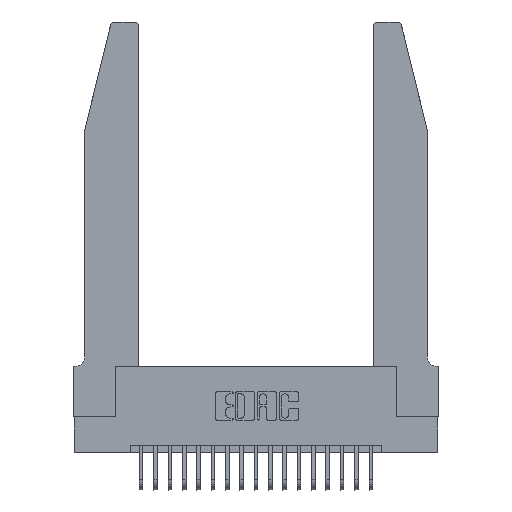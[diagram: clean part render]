
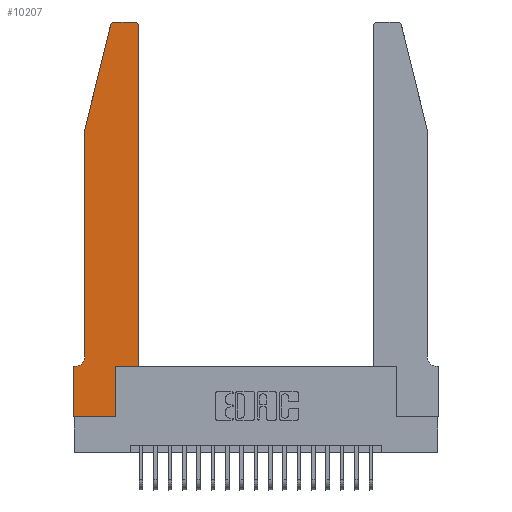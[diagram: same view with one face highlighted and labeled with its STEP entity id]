
A CAD part, top view. The second image highlights one B-rep face of the part: STEP entity #10207.
In plain terms, the highlighted planar face has unit normal (0, 0, 1).
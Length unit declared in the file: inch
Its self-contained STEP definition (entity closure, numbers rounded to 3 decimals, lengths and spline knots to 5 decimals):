
#33 = DIRECTION ( 'NONE',  ( 0., 0., -1. ) ) ;
#140 = LINE ( 'NONE', #16680, #13970 ) ;
#175 = ORIENTED_EDGE ( 'NONE', *, *, #2463, .T. ) ;
#192 = CARTESIAN_POINT ( 'NONE',  ( 0., 0., 0.37 ) ) ;
#350 = VERTEX_POINT ( 'NONE', #192 ) ;
#1004 = DIRECTION ( 'NONE',  ( 1., 0., 0. ) ) ;
#1523 = EDGE_CURVE ( 'NONE', #8714, #16386, #11315, .T. ) ;
#1580 = CARTESIAN_POINT ( 'NONE',  ( 0.0755, 0.42, 0.37 ) ) ;
#1600 = CARTESIAN_POINT ( 'NONE',  ( 0., 0.35, 0.37 ) ) ;
#1772 = VECTOR ( 'NONE', #22418, 39.37008 ) ;
#1988 = ORIENTED_EDGE ( 'NONE', *, *, #7056, .T. ) ;
#2077 = CIRCLE ( 'NONE', #5334, 0.07 ) ;
#2463 = EDGE_CURVE ( 'NONE', #16386, #350, #21253, .T. ) ;
#2477 = VECTOR ( 'NONE', #8777, 39.37008 ) ;
#2504 = ORIENTED_EDGE ( 'NONE', *, *, #20035, .T. ) ;
#3060 = EDGE_CURVE ( 'NONE', #12138, #10161, #10993, .T. ) ;
#3272 = EDGE_CURVE ( 'NONE', #13360, #10950, #6534, .T. ) ;
#3466 = CARTESIAN_POINT ( 'NONE',  ( 0., 0.35, 0.37 ) ) ;
#4598 = CARTESIAN_POINT ( 'NONE',  ( 0.2865, 0.35, 0.37 ) ) ;
#4652 = ORIENTED_EDGE ( 'NONE', *, *, #5797, .T. ) ;
#4899 = VECTOR ( 'NONE', #6230, 39.37008 ) ;
#5225 = ORIENTED_EDGE ( 'NONE', *, *, #17282, .T. ) ;
#5261 = DIRECTION ( 'NONE',  ( 0., 0., 1. ) ) ;
#5334 = AXIS2_PLACEMENT_3D ( 'NONE', #10839, #33, #12690 ) ;
#5691 = DIRECTION ( 'NONE',  ( -1., 0., 0. ) ) ;
#5749 = DIRECTION ( 'NONE',  ( 1., 0., 0. ) ) ;
#5797 = EDGE_CURVE ( 'NONE', #10161, #20009, #22704, .T. ) ;
#5810 = DIRECTION ( 'NONE',  ( 0., 0., 1. ) ) ;
#5892 = EDGE_LOOP ( 'NONE', ( #22410, #4652, #5225, #6139, #2504, #12326, #175, #20078, #11776, #21731, #1988, #7278 ) ) ;
#5941 = CARTESIAN_POINT ( 'NONE',  ( 0.4505, 0.35, 0.37 ) ) ;
#6001 = CARTESIAN_POINT ( 'NONE',  ( 0.0755, 2., 0.37 ) ) ;
#6014 = VECTOR ( 'NONE', #5691, 39.37008 ) ;
#6139 = ORIENTED_EDGE ( 'NONE', *, *, #14868, .T. ) ;
#6230 = DIRECTION ( 'NONE',  ( 0., 1., 0. ) ) ;
#6391 = CARTESIAN_POINT ( 'NONE',  ( 0.2865, 0., 0.37 ) ) ;
#6481 = CARTESIAN_POINT ( 'NONE',  ( 0.4505, 2.72, 0.37 ) ) ;
#6489 = CARTESIAN_POINT ( 'NONE',  ( 0.2605, 2.75, 0.37 ) ) ;
#6495 = VERTEX_POINT ( 'NONE', #6481 ) ;
#6534 = LINE ( 'NONE', #4598, #1772 ) ;
#7056 = EDGE_CURVE ( 'NONE', #10505, #6495, #19098, .T. ) ;
#7063 = VECTOR ( 'NONE', #22277, 39.37008 ) ;
#7187 = LINE ( 'NONE', #15875, #2477 ) ;
#7211 = AXIS2_PLACEMENT_3D ( 'NONE', #16465, #5810, #18267 ) ;
#7278 = ORIENTED_EDGE ( 'NONE', *, *, #14237, .T. ) ;
#7307 = VECTOR ( 'NONE', #5749, 39.37008 ) ;
#7722 = VERTEX_POINT ( 'NONE', #1580 ) ;
#8655 = CARTESIAN_POINT ( 'NONE',  ( 0.0755, 0.35, 0.37 ) ) ;
#8714 = VERTEX_POINT ( 'NONE', #11306 ) ;
#8777 = DIRECTION ( 'NONE',  ( 1., 0., 0. ) ) ;
#9510 = VECTOR ( 'NONE', #18959, 39.37008 ) ;
#10161 = VERTEX_POINT ( 'NONE', #22833 ) ;
#10207 = ADVANCED_FACE ( 'NONE', ( #20591 ), #14140, .T. ) ;
#10505 = VERTEX_POINT ( 'NONE', #5941 ) ;
#10839 = CARTESIAN_POINT ( 'NONE',  ( 0.0055, 0.42, 0.37 ) ) ;
#10887 = EDGE_CURVE ( 'NONE', #350, #13360, #7187, .T. ) ;
#10950 = VERTEX_POINT ( 'NONE', #12583 ) ;
#10993 = LINE ( 'NONE', #6489, #19346 ) ;
#11306 = CARTESIAN_POINT ( 'NONE',  ( 0.0055, 0.35, 0.37 ) ) ;
#11315 = LINE ( 'NONE', #8655, #6014 ) ;
#11752 = DIRECTION ( 'NONE',  ( 0., 0., 1. ) ) ;
#11776 = ORIENTED_EDGE ( 'NONE', *, *, #3272, .T. ) ;
#12138 = VERTEX_POINT ( 'NONE', #13473 ) ;
#12326 = ORIENTED_EDGE ( 'NONE', *, *, #1523, .T. ) ;
#12583 = CARTESIAN_POINT ( 'NONE',  ( 0.2865, 0.35, 0.37 ) ) ;
#12690 = DIRECTION ( 'NONE',  ( -1., 0., 0. ) ) ;
#13360 = VERTEX_POINT ( 'NONE', #6391 ) ;
#13473 = CARTESIAN_POINT ( 'NONE',  ( 0.4205, 2.75, 0.37 ) ) ;
#13708 = AXIS2_PLACEMENT_3D ( 'NONE', #22329, #11752, #1004 ) ;
#13970 = VECTOR ( 'NONE', #18398, 39.37008 ) ;
#14065 = CIRCLE ( 'NONE', #7211, 0.03 ) ;
#14140 = PLANE ( 'NONE',  #15374 ) ;
#14237 = EDGE_CURVE ( 'NONE', #6495, #12138, #14065, .T. ) ;
#14282 = LINE ( 'NONE', #22399, #9510 ) ;
#14563 = EDGE_CURVE ( 'NONE', #10950, #10505, #20403, .T. ) ;
#14868 = EDGE_CURVE ( 'NONE', #20848, #7722, #14282, .T. ) ;
#15374 = AXIS2_PLACEMENT_3D ( 'NONE', #3466, #5261, #17714 ) ;
#15875 = CARTESIAN_POINT ( 'NONE',  ( 0., 0., 0.37 ) ) ;
#16386 = VERTEX_POINT ( 'NONE', #1600 ) ;
#16397 = CARTESIAN_POINT ( 'NONE',  ( 0.4505, 0.35, 0.37 ) ) ;
#16465 = CARTESIAN_POINT ( 'NONE',  ( 0.4205, 2.72, 0.37 ) ) ;
#16680 = CARTESIAN_POINT ( 'NONE',  ( 0.0755, 2., 0.37 ) ) ;
#17282 = EDGE_CURVE ( 'NONE', #20009, #20848, #140, .T. ) ;
#17714 = DIRECTION ( 'NONE',  ( 1., 0., 0. ) ) ;
#18075 = DIRECTION ( 'NONE',  ( -1., 0., 0. ) ) ;
#18267 = DIRECTION ( 'NONE',  ( 1., 0., 0. ) ) ;
#18398 = DIRECTION ( 'NONE',  ( -0.239, -0.971, 0. ) ) ;
#18459 = CARTESIAN_POINT ( 'NONE',  ( 0.25487, 2.72718, 0.37 ) ) ;
#18959 = DIRECTION ( 'NONE',  ( 0., -1., 0. ) ) ;
#19098 = LINE ( 'NONE', #20360, #4899 ) ;
#19346 = VECTOR ( 'NONE', #18075, 39.37008 ) ;
#20009 = VERTEX_POINT ( 'NONE', #18459 ) ;
#20035 = EDGE_CURVE ( 'NONE', #7722, #8714, #2077, .T. ) ;
#20078 = ORIENTED_EDGE ( 'NONE', *, *, #10887, .T. ) ;
#20360 = CARTESIAN_POINT ( 'NONE',  ( 0.4505, 0.35, 0.37 ) ) ;
#20403 = LINE ( 'NONE', #16397, #7307 ) ;
#20533 = CARTESIAN_POINT ( 'NONE',  ( 0., 0., 0.37 ) ) ;
#20591 = FACE_OUTER_BOUND ( 'NONE', #5892, .T. ) ;
#20848 = VERTEX_POINT ( 'NONE', #6001 ) ;
#21253 = LINE ( 'NONE', #20533, #7063 ) ;
#21731 = ORIENTED_EDGE ( 'NONE', *, *, #14563, .T. ) ;
#22277 = DIRECTION ( 'NONE',  ( 0., -1., 0. ) ) ;
#22329 = CARTESIAN_POINT ( 'NONE',  ( 0.284, 2.72, 0.37 ) ) ;
#22399 = CARTESIAN_POINT ( 'NONE',  ( 0.0755, 2., 0.37 ) ) ;
#22410 = ORIENTED_EDGE ( 'NONE', *, *, #3060, .T. ) ;
#22418 = DIRECTION ( 'NONE',  ( 0., 1., 0. ) ) ;
#22704 = CIRCLE ( 'NONE', #13708, 0.03 ) ;
#22833 = CARTESIAN_POINT ( 'NONE',  ( 0.284, 2.75, 0.37 ) ) ;
